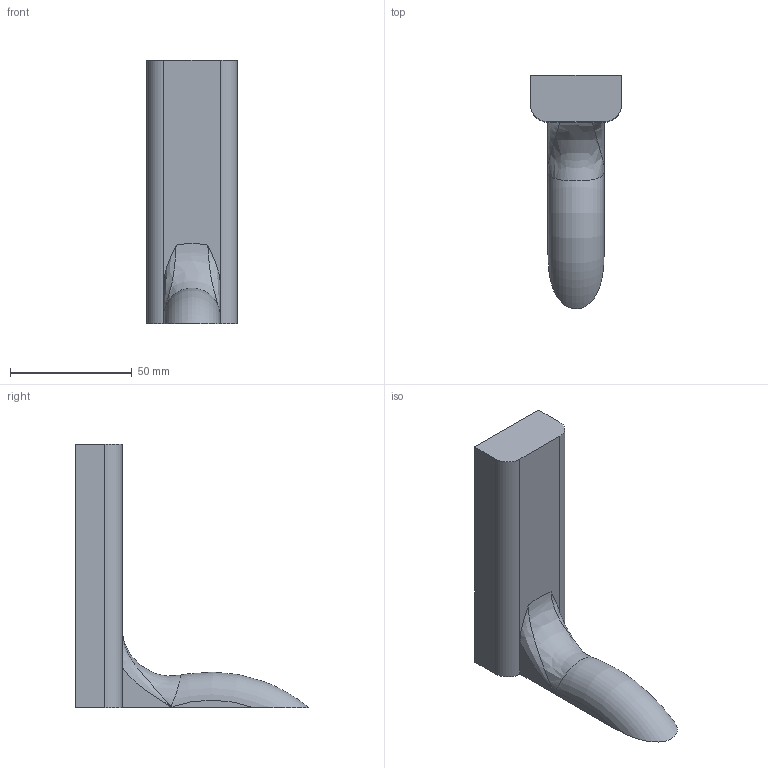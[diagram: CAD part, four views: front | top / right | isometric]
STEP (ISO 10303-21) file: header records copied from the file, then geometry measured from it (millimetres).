
FILE_DESCRIPTION (( 'STEP AP214' ), '1' );
FILE_NAME ('Charon_V3_Pistol_2.STEP', '2013-09-01T16:55:32', ( 'Asher' ), ( '' ), 'SwSTEP 2.0', 'SolidWorks 2013', '' );
FILE_SCHEMA (( 'AUTOMOTIVE_DESIGN' ));
Length unit declared in the file: millimetre
Products named in the file (1): Charon_V3_Pistol_2
Bounding box: 37.13 x 95.6 x 108 mm (x, y, z)
Volume: 92450.9 mm3; surface area: 17403.8 mm2
Topology: 1 solids, 1 shells, 41 faces, 149 edges, 105 vertices
Faces by surface type: sphere 27, plane 8, bspline 3, cylinder 2, torus 1
Entity records: 2098 total; most frequent: CARTESIAN_POINT 1091, DIRECTION 215, ORIENTED_EDGE 174, AXIS2_PLACEMENT_3D 99, EDGE_CURVE 87, VERTEX_POINT 75, EDGE_LOOP 68, CIRCLE 60
